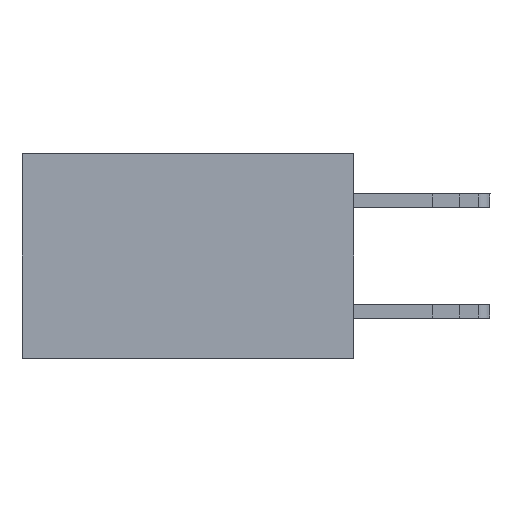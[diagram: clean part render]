
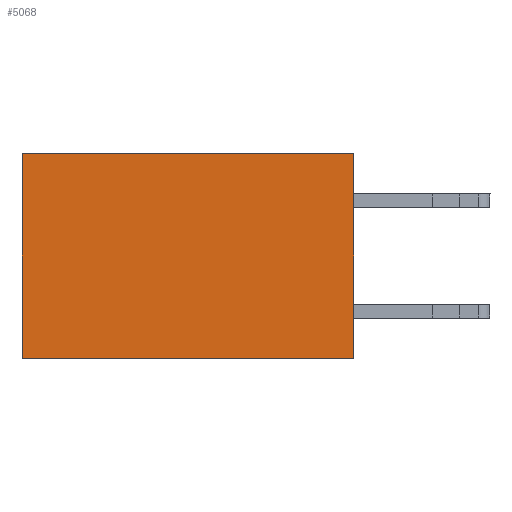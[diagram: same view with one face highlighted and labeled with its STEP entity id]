
A CAD part, left-side view. The second image highlights one B-rep face of the part: STEP entity #5068.
In plain terms, the highlighted planar face has unit normal (-1, 0, 0).
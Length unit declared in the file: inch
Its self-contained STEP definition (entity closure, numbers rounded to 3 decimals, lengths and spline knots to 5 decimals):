
#205 = EDGE_LOOP ( 'NONE', ( #7938, #746, #9269, #19128 ) ) ;
#500 = VECTOR ( 'NONE', #3032, 39.37008 ) ;
#619 = EDGE_CURVE ( 'NONE', #19680, #6590, #12173, .T. ) ;
#746 = ORIENTED_EDGE ( 'NONE', *, *, #18259, .F. ) ;
#2039 = PLANE ( 'NONE',  #14355 ) ;
#3032 = DIRECTION ( 'NONE',  ( 0., 0., -1. ) ) ;
#3714 = DIRECTION ( 'NONE',  ( 0., 0., -1. ) ) ;
#3826 = DIRECTION ( 'NONE',  ( 0., 1., 0. ) ) ;
#3951 = FACE_OUTER_BOUND ( 'NONE', #205, .T. ) ;
#4604 = VERTEX_POINT ( 'NONE', #10540 ) ;
#5068 = ADVANCED_FACE ( 'NONE', ( #3951 ), #2039, .F. ) ;
#5490 = CARTESIAN_POINT ( 'NONE',  ( 0.2875, 0.6, 0. ) ) ;
#5743 = CARTESIAN_POINT ( 'NONE',  ( 0.2875, 0., 0. ) ) ;
#6174 = DIRECTION ( 'NONE',  ( 0., 1., 0. ) ) ;
#6590 = VERTEX_POINT ( 'NONE', #12952 ) ;
#7938 = ORIENTED_EDGE ( 'NONE', *, *, #9107, .T. ) ;
#8008 = VECTOR ( 'NONE', #21556, 39.37008 ) ;
#8936 = LINE ( 'NONE', #5490, #500 ) ;
#9107 = EDGE_CURVE ( 'NONE', #4604, #16779, #8936, .T. ) ;
#9269 = ORIENTED_EDGE ( 'NONE', *, *, #619, .F. ) ;
#10100 = CARTESIAN_POINT ( 'NONE',  ( 0.2875, 0.6, -0.37 ) ) ;
#10270 = CARTESIAN_POINT ( 'NONE',  ( 0.2875, 0., 0. ) ) ;
#10540 = CARTESIAN_POINT ( 'NONE',  ( 0.2875, 0.6, 0. ) ) ;
#10955 = DIRECTION ( 'NONE',  ( 1., 0., 0. ) ) ;
#11744 = LINE ( 'NONE', #20783, #16259 ) ;
#12173 = LINE ( 'NONE', #10270, #8008 ) ;
#12524 = CARTESIAN_POINT ( 'NONE',  ( 0.2875, 0., 0. ) ) ;
#12853 = CARTESIAN_POINT ( 'NONE',  ( 0.2875, 0., 0. ) ) ;
#12952 = CARTESIAN_POINT ( 'NONE',  ( 0.2875, 0., -0.37 ) ) ;
#14355 = AXIS2_PLACEMENT_3D ( 'NONE', #5743, #10955, #3714 ) ;
#14869 = LINE ( 'NONE', #12853, #20040 ) ;
#16259 = VECTOR ( 'NONE', #6174, 39.37008 ) ;
#16779 = VERTEX_POINT ( 'NONE', #10100 ) ;
#17633 = EDGE_CURVE ( 'NONE', #19680, #4604, #14869, .T. ) ;
#18259 = EDGE_CURVE ( 'NONE', #6590, #16779, #11744, .T. ) ;
#19128 = ORIENTED_EDGE ( 'NONE', *, *, #17633, .T. ) ;
#19680 = VERTEX_POINT ( 'NONE', #12524 ) ;
#20040 = VECTOR ( 'NONE', #3826, 39.37008 ) ;
#20783 = CARTESIAN_POINT ( 'NONE',  ( 0.2875, 0., -0.37 ) ) ;
#21556 = DIRECTION ( 'NONE',  ( 0., 0., -1. ) ) ;
